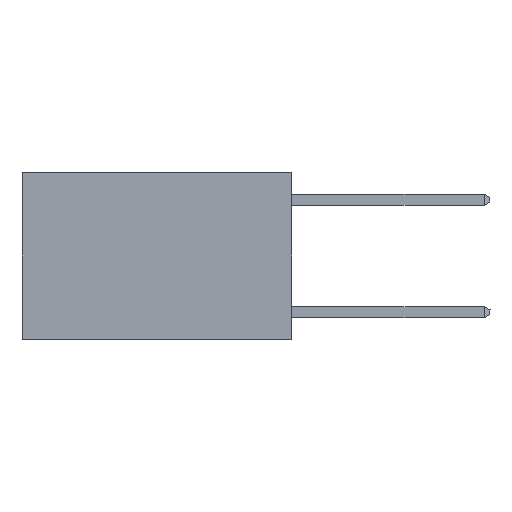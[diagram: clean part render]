
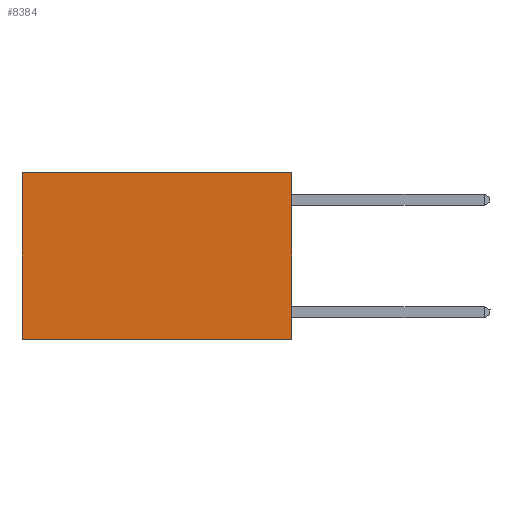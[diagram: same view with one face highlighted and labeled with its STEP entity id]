
A CAD part, left-side view. The second image highlights one B-rep face of the part: STEP entity #8384.
In plain terms, the highlighted planar face has unit normal (-1, 0, 0).
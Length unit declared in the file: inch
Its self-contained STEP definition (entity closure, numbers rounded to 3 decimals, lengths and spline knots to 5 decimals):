
#743 = CARTESIAN_POINT ( 'NONE',  ( 0.2625, 0., 0. ) ) ;
#1546 = DIRECTION ( 'NONE',  ( 0., 0., -1. ) ) ;
#1982 = LINE ( 'NONE', #3904, #9689 ) ;
#2071 = ORIENTED_EDGE ( 'NONE', *, *, #6955, .F. ) ;
#2363 = CARTESIAN_POINT ( 'NONE',  ( 0.2625, 0., 0. ) ) ;
#2396 = EDGE_CURVE ( 'NONE', #8694, #5614, #4314, .T. ) ;
#2482 = VECTOR ( 'NONE', #1546, 39.37008 ) ;
#2507 = VERTEX_POINT ( 'NONE', #3629 ) ;
#3456 = ORIENTED_EDGE ( 'NONE', *, *, #4465, .F. ) ;
#3629 = CARTESIAN_POINT ( 'NONE',  ( 0.2625, 0., -0.37 ) ) ;
#3647 = CARTESIAN_POINT ( 'NONE',  ( 0.2625, 0.6, -0.37 ) ) ;
#3674 = DIRECTION ( 'NONE',  ( 0., 1., 0. ) ) ;
#3884 = FACE_OUTER_BOUND ( 'NONE', #8119, .T. ) ;
#3904 = CARTESIAN_POINT ( 'NONE',  ( 0.2625, 0., 0. ) ) ;
#3939 = DIRECTION ( 'NONE',  ( 0., 1., 0. ) ) ;
#3982 = DIRECTION ( 'NONE',  ( 1., 0., 0. ) ) ;
#3995 = VECTOR ( 'NONE', #3674, 39.37008 ) ;
#4314 = LINE ( 'NONE', #4506, #5803 ) ;
#4390 = DIRECTION ( 'NONE',  ( 0., 0., -1. ) ) ;
#4465 = EDGE_CURVE ( 'NONE', #2507, #5614, #6227, .T. ) ;
#4506 = CARTESIAN_POINT ( 'NONE',  ( 0.2625, 0.6, 0. ) ) ;
#5035 = CARTESIAN_POINT ( 'NONE',  ( 0.2625, 0.6, 0. ) ) ;
#5181 = ORIENTED_EDGE ( 'NONE', *, *, #2396, .T. ) ;
#5614 = VERTEX_POINT ( 'NONE', #3647 ) ;
#5803 = VECTOR ( 'NONE', #4390, 39.37008 ) ;
#6178 = VERTEX_POINT ( 'NONE', #8681 ) ;
#6227 = LINE ( 'NONE', #8125, #3995 ) ;
#6814 = AXIS2_PLACEMENT_3D ( 'NONE', #743, #3982, #9124 ) ;
#6955 = EDGE_CURVE ( 'NONE', #6178, #2507, #8676, .T. ) ;
#8119 = EDGE_LOOP ( 'NONE', ( #5181, #3456, #2071, #8670 ) ) ;
#8125 = CARTESIAN_POINT ( 'NONE',  ( 0.2625, 0., -0.37 ) ) ;
#8384 = ADVANCED_FACE ( 'NONE', ( #3884 ), #8400, .F. ) ;
#8400 = PLANE ( 'NONE',  #6814 ) ;
#8670 = ORIENTED_EDGE ( 'NONE', *, *, #9241, .T. ) ;
#8676 = LINE ( 'NONE', #2363, #2482 ) ;
#8681 = CARTESIAN_POINT ( 'NONE',  ( 0.2625, 0., 0. ) ) ;
#8694 = VERTEX_POINT ( 'NONE', #5035 ) ;
#9124 = DIRECTION ( 'NONE',  ( 0., 0., -1. ) ) ;
#9241 = EDGE_CURVE ( 'NONE', #6178, #8694, #1982, .T. ) ;
#9689 = VECTOR ( 'NONE', #3939, 39.37008 ) ;
